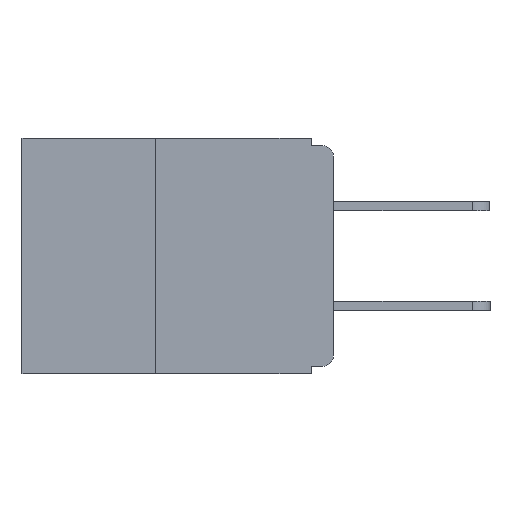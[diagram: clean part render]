
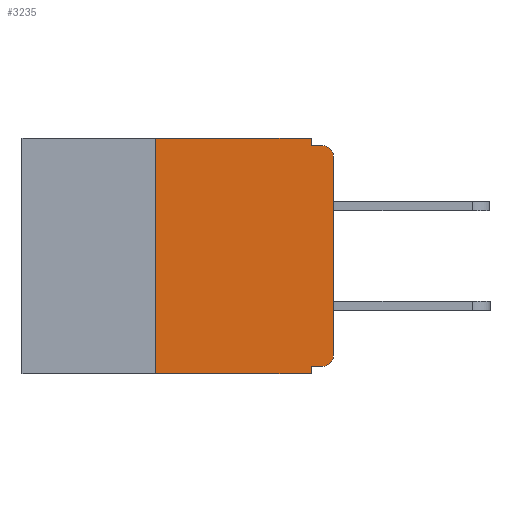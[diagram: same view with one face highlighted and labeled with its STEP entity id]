
A CAD part, left-side view. The second image highlights one B-rep face of the part: STEP entity #3235.
In plain terms, the highlighted planar face has unit normal (-1, 0, 0).
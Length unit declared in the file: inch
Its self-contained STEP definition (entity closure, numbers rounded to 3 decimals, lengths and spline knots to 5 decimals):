
#73 = CARTESIAN_POINT ( 'NONE',  ( 0., 0.015, -0.01 ) ) ;
#572 = EDGE_CURVE ( 'NONE', #2027, #9534, #8769, .T. ) ;
#585 = VERTEX_POINT ( 'NONE', #1824 ) ;
#711 = DIRECTION ( 'NONE',  ( 0., 1., 0. ) ) ;
#1191 = VECTOR ( 'NONE', #7475, 39.37008 ) ;
#1611 = CARTESIAN_POINT ( 'NONE',  ( 0., 0., -0.32 ) ) ;
#1661 = CARTESIAN_POINT ( 'NONE',  ( 0., 0.031, 0. ) ) ;
#1748 = CARTESIAN_POINT ( 'NONE',  ( 0., 0.25, -0.33 ) ) ;
#1824 = CARTESIAN_POINT ( 'NONE',  ( 0., 0.25, -0.33 ) ) ;
#2027 = VERTEX_POINT ( 'NONE', #5252 ) ;
#2145 = PLANE ( 'NONE',  #6441 ) ;
#2188 = CARTESIAN_POINT ( 'NONE',  ( 0., 0., -0.305 ) ) ;
#2510 = ORIENTED_EDGE ( 'NONE', *, *, #7687, .F. ) ;
#2575 = LINE ( 'NONE', #12253, #7492 ) ;
#3092 = ORIENTED_EDGE ( 'NONE', *, *, #572, .F. ) ;
#3235 = ADVANCED_FACE ( 'NONE', ( #13287 ), #2145, .F. ) ;
#3247 = EDGE_CURVE ( 'NONE', #13708, #13884, #3826, .T. ) ;
#3271 = VECTOR ( 'NONE', #4834, 39.37008 ) ;
#3364 = CARTESIAN_POINT ( 'NONE',  ( 0., 0., 0. ) ) ;
#3498 = CARTESIAN_POINT ( 'NONE',  ( 0., 0.437, 0. ) ) ;
#3565 = ORIENTED_EDGE ( 'NONE', *, *, #5867, .T. ) ;
#3803 = AXIS2_PLACEMENT_3D ( 'NONE', #6446, #14647, #7638 ) ;
#3826 = LINE ( 'NONE', #3364, #7073 ) ;
#4094 = DIRECTION ( 'NONE',  ( 0., 0., 1. ) ) ;
#4438 = LINE ( 'NONE', #13304, #1191 ) ;
#4478 = CIRCLE ( 'NONE', #11939, 0.015 ) ;
#4829 = VERTEX_POINT ( 'NONE', #1661 ) ;
#4834 = DIRECTION ( 'NONE',  ( 0., 0., -1. ) ) ;
#4975 = VECTOR ( 'NONE', #11820, 39.37008 ) ;
#5007 = CARTESIAN_POINT ( 'NONE',  ( 0., 0., -0.025 ) ) ;
#5053 = CARTESIAN_POINT ( 'NONE',  ( 0., 0.031, -0.01 ) ) ;
#5199 = DIRECTION ( 'NONE',  ( 0., 0., -1. ) ) ;
#5252 = CARTESIAN_POINT ( 'NONE',  ( 0., 0.015, -0.32 ) ) ;
#5541 = ORIENTED_EDGE ( 'NONE', *, *, #13034, .F. ) ;
#5562 = EDGE_CURVE ( 'NONE', #585, #13906, #9315, .T. ) ;
#5867 = EDGE_CURVE ( 'NONE', #2027, #13708, #4478, .T. ) ;
#6028 = VECTOR ( 'NONE', #711, 39.37008 ) ;
#6441 = AXIS2_PLACEMENT_3D ( 'NONE', #6932, #9067, #9517 ) ;
#6446 = CARTESIAN_POINT ( 'NONE',  ( 0., 0.015, -0.025 ) ) ;
#6517 = LINE ( 'NONE', #8374, #3271 ) ;
#6816 = EDGE_LOOP ( 'NONE', ( #14849, #12984, #2510, #5541, #8279, #14463, #12783, #7609, #3092, #3565 ) ) ;
#6932 = CARTESIAN_POINT ( 'NONE',  ( 0., 0.437, 0. ) ) ;
#7073 = VECTOR ( 'NONE', #4094, 39.37008 ) ;
#7273 = DIRECTION ( 'NONE',  ( -1., 0., 0. ) ) ;
#7475 = DIRECTION ( 'NONE',  ( 0., -1., 0. ) ) ;
#7492 = VECTOR ( 'NONE', #5199, 39.37008 ) ;
#7609 = ORIENTED_EDGE ( 'NONE', *, *, #11469, .F. ) ;
#7638 = DIRECTION ( 'NONE',  ( 0., 0., -1. ) ) ;
#7687 = EDGE_CURVE ( 'NONE', #12529, #9046, #13470, .T. ) ;
#7919 = CIRCLE ( 'NONE', #3803, 0.015 ) ;
#8279 = ORIENTED_EDGE ( 'NONE', *, *, #14340, .F. ) ;
#8374 = CARTESIAN_POINT ( 'NONE',  ( 0., 0.031, 0. ) ) ;
#8594 = CARTESIAN_POINT ( 'NONE',  ( 0., 0.25, 0. ) ) ;
#8769 = LINE ( 'NONE', #1611, #6028 ) ;
#9046 = VERTEX_POINT ( 'NONE', #73 ) ;
#9067 = DIRECTION ( 'NONE',  ( 1., 0., 0. ) ) ;
#9309 = CARTESIAN_POINT ( 'NONE',  ( 0., 0., -0.01 ) ) ;
#9315 = LINE ( 'NONE', #1748, #12431 ) ;
#9401 = VERTEX_POINT ( 'NONE', #12700 ) ;
#9465 = CARTESIAN_POINT ( 'NONE',  ( 0., 0.031, -0.32 ) ) ;
#9517 = DIRECTION ( 'NONE',  ( 0., 0., -1. ) ) ;
#9534 = VERTEX_POINT ( 'NONE', #9465 ) ;
#9777 = EDGE_CURVE ( 'NONE', #13884, #9046, #7919, .T. ) ;
#11250 = LINE ( 'NONE', #3498, #4975 ) ;
#11469 = EDGE_CURVE ( 'NONE', #9534, #9401, #2575, .T. ) ;
#11820 = DIRECTION ( 'NONE',  ( 0., -1., 0. ) ) ;
#11939 = AXIS2_PLACEMENT_3D ( 'NONE', #14295, #7273, #13394 ) ;
#12253 = CARTESIAN_POINT ( 'NONE',  ( 0., 0.031, -0.33 ) ) ;
#12431 = VECTOR ( 'NONE', #13672, 39.37008 ) ;
#12529 = VERTEX_POINT ( 'NONE', #5053 ) ;
#12544 = EDGE_CURVE ( 'NONE', #585, #9401, #4438, .T. ) ;
#12700 = CARTESIAN_POINT ( 'NONE',  ( 0., 0.031, -0.33 ) ) ;
#12783 = ORIENTED_EDGE ( 'NONE', *, *, #12544, .T. ) ;
#12984 = ORIENTED_EDGE ( 'NONE', *, *, #9777, .T. ) ;
#13034 = EDGE_CURVE ( 'NONE', #4829, #12529, #6517, .T. ) ;
#13111 = VECTOR ( 'NONE', #15130, 39.37008 ) ;
#13287 = FACE_OUTER_BOUND ( 'NONE', #6816, .T. ) ;
#13304 = CARTESIAN_POINT ( 'NONE',  ( 0., 0.437, -0.33 ) ) ;
#13394 = DIRECTION ( 'NONE',  ( 0., 0., -1. ) ) ;
#13470 = LINE ( 'NONE', #9309, #13111 ) ;
#13672 = DIRECTION ( 'NONE',  ( 0., 0., 1. ) ) ;
#13708 = VERTEX_POINT ( 'NONE', #2188 ) ;
#13884 = VERTEX_POINT ( 'NONE', #5007 ) ;
#13906 = VERTEX_POINT ( 'NONE', #8594 ) ;
#14295 = CARTESIAN_POINT ( 'NONE',  ( 0., 0.015, -0.305 ) ) ;
#14340 = EDGE_CURVE ( 'NONE', #13906, #4829, #11250, .T. ) ;
#14463 = ORIENTED_EDGE ( 'NONE', *, *, #5562, .F. ) ;
#14647 = DIRECTION ( 'NONE',  ( -1., 0., 0. ) ) ;
#14849 = ORIENTED_EDGE ( 'NONE', *, *, #3247, .T. ) ;
#15130 = DIRECTION ( 'NONE',  ( 0., -1., 0. ) ) ;
